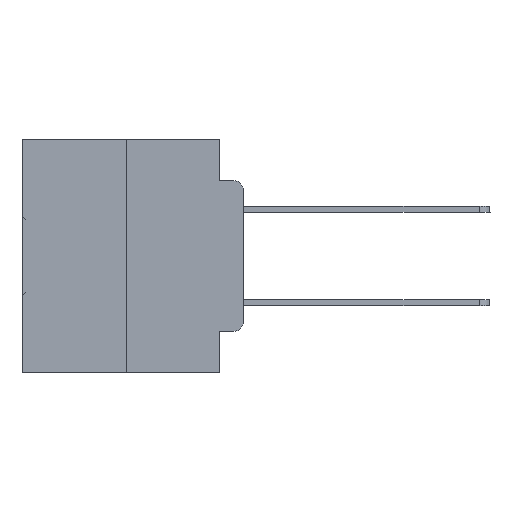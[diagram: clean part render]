
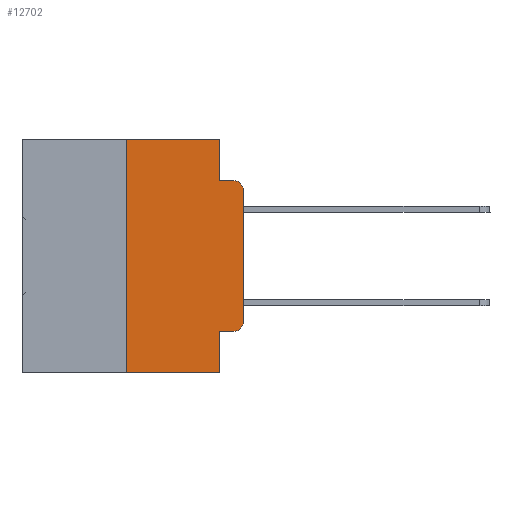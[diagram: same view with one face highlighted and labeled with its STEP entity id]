
A CAD part, left-side view. The second image highlights one B-rep face of the part: STEP entity #12702.
In plain terms, the highlighted planar face has unit normal (-1, 0, 0).
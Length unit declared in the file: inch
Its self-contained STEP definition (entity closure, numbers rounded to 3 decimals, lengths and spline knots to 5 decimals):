
#626 = VERTEX_POINT ( 'NONE', #8055 ) ;
#652 = VECTOR ( 'NONE', #21078, 39.37008 ) ;
#833 = LINE ( 'NONE', #9848, #14653 ) ;
#1069 = VECTOR ( 'NONE', #18473, 39.37008 ) ;
#1761 = DIRECTION ( 'NONE',  ( 0., -1., 0. ) ) ;
#1907 = VERTEX_POINT ( 'NONE', #20934 ) ;
#2070 = ORIENTED_EDGE ( 'NONE', *, *, #5022, .T. ) ;
#2888 = CARTESIAN_POINT ( 'NONE',  ( 0., 0.473, 0. ) ) ;
#3413 = LINE ( 'NONE', #2888, #31036 ) ;
#3585 = LINE ( 'NONE', #18127, #1069 ) ;
#3718 = EDGE_CURVE ( 'NONE', #29304, #32325, #10796, .T. ) ;
#4171 = PLANE ( 'NONE',  #12378 ) ;
#4628 = ORIENTED_EDGE ( 'NONE', *, *, #27259, .F. ) ;
#4652 = ORIENTED_EDGE ( 'NONE', *, *, #29354, .F. ) ;
#5022 = EDGE_CURVE ( 'NONE', #6038, #29304, #3585, .T. ) ;
#5054 = EDGE_CURVE ( 'NONE', #20504, #9196, #12375, .T. ) ;
#6038 = VERTEX_POINT ( 'NONE', #29411 ) ;
#6150 = VECTOR ( 'NONE', #26130, 39.37008 ) ;
#6761 = LINE ( 'NONE', #20362, #19344 ) ;
#6837 = CARTESIAN_POINT ( 'NONE',  ( 0., 0.473, 0. ) ) ;
#6963 = DIRECTION ( 'NONE',  ( 1., 0., 0. ) ) ;
#7101 = CARTESIAN_POINT ( 'NONE',  ( 0., 0.02, -0.1085 ) ) ;
#7271 = ORIENTED_EDGE ( 'NONE', *, *, #3718, .T. ) ;
#8055 = CARTESIAN_POINT ( 'NONE',  ( 0., 0., -0.1085 ) ) ;
#8345 = DIRECTION ( 'NONE',  ( 0., 0., -1. ) ) ;
#8413 = CARTESIAN_POINT ( 'NONE',  ( 0., 0.051, -0.0885 ) ) ;
#9196 = VERTEX_POINT ( 'NONE', #17082 ) ;
#9437 = DIRECTION ( 'NONE',  ( 0., 0., -1. ) ) ;
#9672 = ORIENTED_EDGE ( 'NONE', *, *, #5054, .F. ) ;
#9787 = ORIENTED_EDGE ( 'NONE', *, *, #30157, .F. ) ;
#9848 = CARTESIAN_POINT ( 'NONE',  ( 0., 0.051, 0. ) ) ;
#10341 = DIRECTION ( 'NONE',  ( 0., 0., 1. ) ) ;
#10796 = CIRCLE ( 'NONE', #32962, 0.02 ) ;
#11201 = AXIS2_PLACEMENT_3D ( 'NONE', #7101, #17603, #9437 ) ;
#12375 = LINE ( 'NONE', #31942, #652 ) ;
#12378 = AXIS2_PLACEMENT_3D ( 'NONE', #6837, #6963, #28267 ) ;
#12702 = ADVANCED_FACE ( 'NONE', ( #16296 ), #4171, .F. ) ;
#12900 = CARTESIAN_POINT ( 'NONE',  ( 0., 0.25, 0. ) ) ;
#13026 = VERTEX_POINT ( 'NONE', #18535 ) ;
#14399 = EDGE_CURVE ( 'NONE', #1907, #30677, #6761, .T. ) ;
#14653 = VECTOR ( 'NONE', #15226, 39.37008 ) ;
#15083 = CARTESIAN_POINT ( 'NONE',  ( 0., 0.051, -0.5 ) ) ;
#15226 = DIRECTION ( 'NONE',  ( 0., 0., -1. ) ) ;
#15350 = CARTESIAN_POINT ( 'NONE',  ( 0., 0.051, 0. ) ) ;
#15556 = ORIENTED_EDGE ( 'NONE', *, *, #14399, .T. ) ;
#16296 = FACE_OUTER_BOUND ( 'NONE', #26830, .T. ) ;
#17082 = CARTESIAN_POINT ( 'NONE',  ( 0., 0.02, -0.0885 ) ) ;
#17603 = DIRECTION ( 'NONE',  ( -1., 0., 0. ) ) ;
#17825 = ORIENTED_EDGE ( 'NONE', *, *, #20955, .T. ) ;
#18127 = CARTESIAN_POINT ( 'NONE',  ( 0., 0.051, -0.4115 ) ) ;
#18162 = CARTESIAN_POINT ( 'NONE',  ( 0., 0., 0. ) ) ;
#18473 = DIRECTION ( 'NONE',  ( 0., -1., 0. ) ) ;
#18535 = CARTESIAN_POINT ( 'NONE',  ( 0., 0.25, 0. ) ) ;
#19182 = DIRECTION ( 'NONE',  ( -1., 0., 0. ) ) ;
#19344 = VECTOR ( 'NONE', #1761, 39.37008 ) ;
#19454 = CIRCLE ( 'NONE', #11201, 0.02 ) ;
#20362 = CARTESIAN_POINT ( 'NONE',  ( 0., 0.473, -0.5 ) ) ;
#20419 = EDGE_CURVE ( 'NONE', #13026, #33404, #3413, .T. ) ;
#20456 = LINE ( 'NONE', #15350, #32162 ) ;
#20504 = VERTEX_POINT ( 'NONE', #8413 ) ;
#20934 = CARTESIAN_POINT ( 'NONE',  ( 0., 0.25, -0.5 ) ) ;
#20945 = LINE ( 'NONE', #18162, #27236 ) ;
#20955 = EDGE_CURVE ( 'NONE', #32325, #626, #20945, .T. ) ;
#21078 = DIRECTION ( 'NONE',  ( 0., -1., 0. ) ) ;
#22971 = CARTESIAN_POINT ( 'NONE',  ( 0., 0.02, -0.4115 ) ) ;
#23704 = DIRECTION ( 'NONE',  ( 0., -1., 0. ) ) ;
#25161 = CARTESIAN_POINT ( 'NONE',  ( 0., 0., -0.3915 ) ) ;
#26130 = DIRECTION ( 'NONE',  ( 0., 0., 1. ) ) ;
#26830 = EDGE_LOOP ( 'NONE', ( #17825, #29089, #9672, #9787, #30513, #4628, #15556, #4652, #2070, #7271 ) ) ;
#27236 = VECTOR ( 'NONE', #10341, 39.37008 ) ;
#27259 = EDGE_CURVE ( 'NONE', #1907, #13026, #27515, .T. ) ;
#27515 = LINE ( 'NONE', #12900, #6150 ) ;
#28267 = DIRECTION ( 'NONE',  ( 0., 0., -1. ) ) ;
#28692 = EDGE_CURVE ( 'NONE', #626, #9196, #19454, .T. ) ;
#29089 = ORIENTED_EDGE ( 'NONE', *, *, #28692, .T. ) ;
#29304 = VERTEX_POINT ( 'NONE', #22971 ) ;
#29354 = EDGE_CURVE ( 'NONE', #6038, #30677, #833, .T. ) ;
#29411 = CARTESIAN_POINT ( 'NONE',  ( 0., 0.051, -0.4115 ) ) ;
#29473 = DIRECTION ( 'NONE',  ( 0., 0., -1. ) ) ;
#30157 = EDGE_CURVE ( 'NONE', #33404, #20504, #20456, .T. ) ;
#30513 = ORIENTED_EDGE ( 'NONE', *, *, #20419, .F. ) ;
#30677 = VERTEX_POINT ( 'NONE', #15083 ) ;
#31036 = VECTOR ( 'NONE', #23704, 39.37008 ) ;
#31942 = CARTESIAN_POINT ( 'NONE',  ( 0., 0.051, -0.0885 ) ) ;
#32162 = VECTOR ( 'NONE', #29473, 39.37008 ) ;
#32325 = VERTEX_POINT ( 'NONE', #25161 ) ;
#32531 = CARTESIAN_POINT ( 'NONE',  ( 0., 0.02, -0.3915 ) ) ;
#32962 = AXIS2_PLACEMENT_3D ( 'NONE', #32531, #19182, #8345 ) ;
#33404 = VERTEX_POINT ( 'NONE', #33728 ) ;
#33728 = CARTESIAN_POINT ( 'NONE',  ( 0., 0.051, 0. ) ) ;
